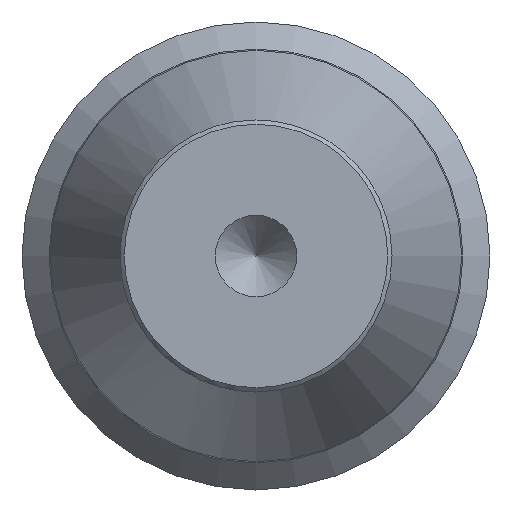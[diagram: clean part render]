
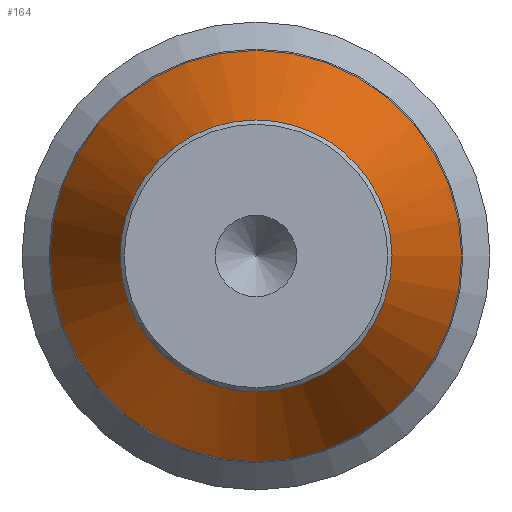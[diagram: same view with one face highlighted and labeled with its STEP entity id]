
A CAD part, left-side view. The second image highlights one B-rep face of the part: STEP entity #164.
In plain terms, the highlighted free-form (B-spline) face has degree [1, 13] with [2, 14] control points.
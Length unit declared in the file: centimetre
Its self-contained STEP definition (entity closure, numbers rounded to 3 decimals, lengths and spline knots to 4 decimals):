
#13=B_SPLINE_CURVE_WITH_KNOTS($,13,(#315,#316,#317,#318,#319,#320,#321,
#322,#323,#324,#325,#326,#327,#328),.UNSPECIFIED.,.F.,.F.,(14,14),(26.2323,
52.4646),.UNSPECIFIED.);
#14=B_SPLINE_CURVE_WITH_KNOTS($,13,(#329,#330,#331,#332,#333,#334,#335,
#336,#337,#338,#339,#340,#341,#342),.UNSPECIFIED.,.F.,.F.,(14,14),(0.,
26.2323),.UNSPECIFIED.);
#15=LINE($,#313,#16);
#16=VECTOR($,#244,0.7391);
#17=B_SPLINE_SURFACE_WITH_KNOTS($,1,13,((#284,#285,#286,#287,#288,#289,
#290,#291,#292,#293,#294,#295,#296,#297),(#298,#299,#300,#301,#302,#303,
#304,#305,#306,#307,#308,#309,#310,#311)),.UNSPECIFIED.,.F.,.T.,.F.,(2,
2),(14,14),(-0.0008,52.4646),(0.,
52.4646),.UNSPECIFIED.);
#52=FACE_OUTER_BOUND($,#76,.T.);
#76=EDGE_LOOP($,(#142,#143,#144,#145,#146));
#81=CIRCLE($,#173,0.835);
#93=VERTEX_POINT($,#254);
#103=VERTEX_POINT($,#312);
#104=VERTEX_POINT($,#314);
#107=EDGE_CURVE($,#93,#93,#81,.T.);
#117=EDGE_CURVE($,#93,#103,#15,.T.);
#118=EDGE_CURVE($,#104,#103,#13,.T.);
#119=EDGE_CURVE($,#103,#104,#14,.T.);
#142=ORIENTED_EDGE($,*,*,#117,.F.);
#143=ORIENTED_EDGE($,*,*,#107,.T.);
#144=ORIENTED_EDGE($,*,*,#117,.T.);
#145=ORIENTED_EDGE($,*,*,#118,.F.);
#146=ORIENTED_EDGE($,*,*,#119,.F.);
#164=ADVANCED_FACE($,(#52),#17,.F.);
#173=AXIS2_PLACEMENT_3D($,#255,#204,#205);
#204=DIRECTION('center_axis',(-1.,0.,0.));
#205=DIRECTION('ref_axis',(0.,-0.588,0.809));
#244=DIRECTION($,(-0.924,0.,-0.383));
#254=CARTESIAN_POINT('',(-10.721,4.6595,0.9031));
#255=CARTESIAN_POINT('Origin',(-10.721,4.6595,0.0681));
#284=CARTESIAN_POINT('Ctrl Pts',(-10.7209,4.6595,0.9031));
#285=CARTESIAN_POINT('Ctrl Pts',(-10.7209,5.0572,0.9031));
#286=CARTESIAN_POINT('Ctrl Pts',(-10.7209,5.4641,0.6976));
#287=CARTESIAN_POINT('Ctrl Pts',(-10.7209,5.7551,0.2745));
#288=CARTESIAN_POINT('Ctrl Pts',(-10.7209,5.7998,-0.3076));
#289=CARTESIAN_POINT('Ctrl Pts',(-10.7209,5.4896,-0.8105));
#290=CARTESIAN_POINT('Ctrl Pts',(-10.7209,5.0369,-1.1793));
#291=CARTESIAN_POINT('Ctrl Pts',(-10.7209,4.282,-1.1793));
#292=CARTESIAN_POINT('Ctrl Pts',(-10.7209,3.8293,-0.8105));
#293=CARTESIAN_POINT('Ctrl Pts',(-10.7209,3.5192,-0.3076));
#294=CARTESIAN_POINT('Ctrl Pts',(-10.7209,3.5639,0.2745));
#295=CARTESIAN_POINT('Ctrl Pts',(-10.7209,3.8548,0.6976));
#296=CARTESIAN_POINT('Ctrl Pts',(-10.7209,4.2617,0.9031));
#297=CARTESIAN_POINT('Ctrl Pts',(-10.7209,4.6595,0.9031));
#298=CARTESIAN_POINT('Ctrl Pts',(-11.4038,4.6595,0.6203));
#299=CARTESIAN_POINT('Ctrl Pts',(-11.4038,4.9225,0.6203));
#300=CARTESIAN_POINT('Ctrl Pts',(-11.4038,5.1915,0.4843));
#301=CARTESIAN_POINT('Ctrl Pts',(-11.4038,5.3839,0.2046));
#302=CARTESIAN_POINT('Ctrl Pts',(-11.4038,5.4135,-0.1803));
#303=CARTESIAN_POINT('Ctrl Pts',(-11.4038,5.2084,-0.5129));
#304=CARTESIAN_POINT('Ctrl Pts',(-11.4038,4.9091,-0.7568));
#305=CARTESIAN_POINT('Ctrl Pts',(-11.4038,4.4099,-0.7568));
#306=CARTESIAN_POINT('Ctrl Pts',(-11.4038,4.1105,-0.5129));
#307=CARTESIAN_POINT('Ctrl Pts',(-11.4038,3.9054,-0.1803));
#308=CARTESIAN_POINT('Ctrl Pts',(-11.4038,3.935,0.2046));
#309=CARTESIAN_POINT('Ctrl Pts',(-11.4038,4.1274,0.4843));
#310=CARTESIAN_POINT('Ctrl Pts',(-11.4038,4.3965,0.6203));
#311=CARTESIAN_POINT('Ctrl Pts',(-11.4038,4.6595,0.6203));
#312=CARTESIAN_POINT('',(-11.4038,4.6595,0.6203));
#313=CARTESIAN_POINT($,(-10.721,4.6595,0.9031));
#314=CARTESIAN_POINT('',(-11.4038,4.6595,-0.484));
#315=CARTESIAN_POINT('Ctrl Pts',(-11.4038,4.6595,-0.484));
#316=CARTESIAN_POINT('Ctrl Pts',(-11.4038,4.526,-0.484));
#317=CARTESIAN_POINT('Ctrl Pts',(-11.4038,4.3926,-0.4491));
#318=CARTESIAN_POINT('Ctrl Pts',(-11.4038,4.2691,-0.3793));
#319=CARTESIAN_POINT('Ctrl Pts',(-11.4038,4.1656,-0.2776));
#320=CARTESIAN_POINT('Ctrl Pts',(-11.4038,4.0909,-0.1504));
#321=CARTESIAN_POINT('Ctrl Pts',(-11.4038,4.0517,-0.0066));
#322=CARTESIAN_POINT('Ctrl Pts',(-11.4038,4.0516,0.1431));
#323=CARTESIAN_POINT('Ctrl Pts',(-11.4038,4.0907,0.2874));
#324=CARTESIAN_POINT('Ctrl Pts',(-11.4038,4.1659,0.4153));
#325=CARTESIAN_POINT('Ctrl Pts',(-11.4038,4.2707,0.5173));
#326=CARTESIAN_POINT('Ctrl Pts',(-11.4038,4.3949,0.5863));
#327=CARTESIAN_POINT('Ctrl Pts',(-11.4038,4.528,0.6203));
#328=CARTESIAN_POINT('Ctrl Pts',(-11.4038,4.6595,0.6203));
#329=CARTESIAN_POINT('Ctrl Pts',(-11.4038,4.6595,0.6203));
#330=CARTESIAN_POINT('Ctrl Pts',(-11.4038,4.791,0.6203));
#331=CARTESIAN_POINT('Ctrl Pts',(-11.4038,4.924,0.5863));
#332=CARTESIAN_POINT('Ctrl Pts',(-11.4038,5.0482,0.5173));
#333=CARTESIAN_POINT('Ctrl Pts',(-11.4038,5.153,0.4153));
#334=CARTESIAN_POINT('Ctrl Pts',(-11.4038,5.2282,0.2874));
#335=CARTESIAN_POINT('Ctrl Pts',(-11.4038,5.2673,0.1431));
#336=CARTESIAN_POINT('Ctrl Pts',(-11.4038,5.2672,-0.0066));
#337=CARTESIAN_POINT('Ctrl Pts',(-11.4038,5.228,-0.1504));
#338=CARTESIAN_POINT('Ctrl Pts',(-11.4038,5.1533,-0.2776));
#339=CARTESIAN_POINT('Ctrl Pts',(-11.4038,5.0498,-0.3793));
#340=CARTESIAN_POINT('Ctrl Pts',(-11.4038,4.9263,-0.4491));
#341=CARTESIAN_POINT('Ctrl Pts',(-11.4038,4.7929,-0.484));
#342=CARTESIAN_POINT('Ctrl Pts',(-11.4038,4.6595,-0.484));
